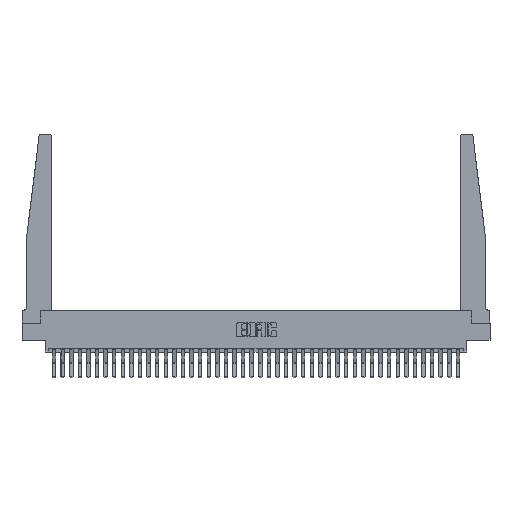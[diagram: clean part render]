
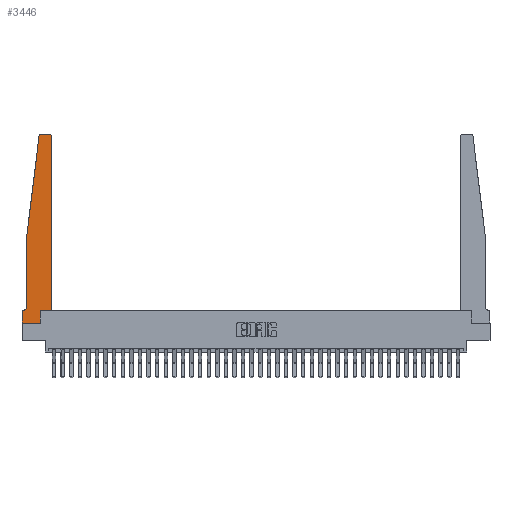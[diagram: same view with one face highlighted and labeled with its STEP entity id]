
A CAD part, top view. The second image highlights one B-rep face of the part: STEP entity #3446.
In plain terms, the highlighted planar face has unit normal (0, 0, 1).
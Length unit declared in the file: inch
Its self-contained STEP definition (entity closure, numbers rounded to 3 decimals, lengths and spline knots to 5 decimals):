
#540 = CARTESIAN_POINT ( 'NONE',  ( 0.27653, 2.75, 0.37 ) ) ;
#650 = ORIENTED_EDGE ( 'NONE', *, *, #20434, .T. ) ;
#983 = CARTESIAN_POINT ( 'NONE',  ( 0.25, 2.75, 0.37 ) ) ;
#1507 = LINE ( 'NONE', #15884, #22641 ) ;
#3208 = VERTEX_POINT ( 'NONE', #31765 ) ;
#3403 = VERTEX_POINT ( 'NONE', #35305 ) ;
#3446 = ADVANCED_FACE ( 'NONE', ( #24439 ), #34013, .T. ) ;
#3788 = LINE ( 'NONE', #25565, #17601 ) ;
#3988 = DIRECTION ( 'NONE',  ( 0., 1., 0. ) ) ;
#4056 = VERTEX_POINT ( 'NONE', #32637 ) ;
#4245 = DIRECTION ( 'NONE',  ( 0., 0., 1. ) ) ;
#4459 = EDGE_LOOP ( 'NONE', ( #25759, #8160, #12875, #28646, #28439, #14412, #33113, #16651, #10961, #32557, #8460, #650 ) ) ;
#5536 = EDGE_CURVE ( 'NONE', #4056, #25676, #3788, .T. ) ;
#5599 = DIRECTION ( 'NONE',  ( 1., 0., 0. ) ) ;
#6557 = LINE ( 'NONE', #22729, #34736 ) ;
#6653 = CARTESIAN_POINT ( 'NONE',  ( 0.395, 2.75, 0.37 ) ) ;
#6776 = EDGE_CURVE ( 'NONE', #15526, #3403, #23460, .T. ) ;
#6938 = VECTOR ( 'NONE', #19695, 39.37008 ) ;
#7162 = EDGE_CURVE ( 'NONE', #23891, #4056, #19611, .T. ) ;
#7681 = DIRECTION ( 'NONE',  ( 0., -1., 0. ) ) ;
#8160 = ORIENTED_EDGE ( 'NONE', *, *, #6776, .T. ) ;
#8460 = ORIENTED_EDGE ( 'NONE', *, *, #5536, .T. ) ;
#10553 = CARTESIAN_POINT ( 'NONE',  ( 0.395, 2.72, 0.37 ) ) ;
#10701 = VECTOR ( 'NONE', #24409, 39.37008 ) ;
#10736 = LINE ( 'NONE', #14856, #15462 ) ;
#10961 = ORIENTED_EDGE ( 'NONE', *, *, #34672, .T. ) ;
#11161 = EDGE_CURVE ( 'NONE', #18633, #24408, #19381, .T. ) ;
#11274 = DIRECTION ( 'NONE',  ( 0., 0., -1. ) ) ;
#11340 = DIRECTION ( 'NONE',  ( 1., 0., 0. ) ) ;
#11742 = CARTESIAN_POINT ( 'NONE',  ( 0.2605, 0., 0.37 ) ) ;
#11994 = DIRECTION ( 'NONE',  ( -1., 0., 0. ) ) ;
#12469 = EDGE_CURVE ( 'NONE', #23445, #20112, #1507, .T. ) ;
#12875 = ORIENTED_EDGE ( 'NONE', *, *, #27185, .T. ) ;
#12993 = VECTOR ( 'NONE', #19134, 39.37008 ) ;
#13334 = DIRECTION ( 'NONE',  ( 1., 0., 0. ) ) ;
#13800 = CARTESIAN_POINT ( 'NONE',  ( 0., 0.1875, 0.37 ) ) ;
#14283 = LINE ( 'NONE', #16962, #6938 ) ;
#14360 = AXIS2_PLACEMENT_3D ( 'NONE', #10553, #29613, #13334 ) ;
#14412 = ORIENTED_EDGE ( 'NONE', *, *, #16298, .T. ) ;
#14856 = CARTESIAN_POINT ( 'NONE',  ( 0.2605, 0.18, 0.37 ) ) ;
#15130 = AXIS2_PLACEMENT_3D ( 'NONE', #27582, #11274, #30314 ) ;
#15462 = VECTOR ( 'NONE', #3988, 39.37008 ) ;
#15526 = VERTEX_POINT ( 'NONE', #540 ) ;
#15884 = CARTESIAN_POINT ( 'NONE',  ( 0.065, 1.25, 0.37 ) ) ;
#16215 = CARTESIAN_POINT ( 'NONE',  ( 0.065, 1.25, 0.37 ) ) ;
#16298 = EDGE_CURVE ( 'NONE', #3208, #18633, #6557, .T. ) ;
#16651 = ORIENTED_EDGE ( 'NONE', *, *, #25173, .T. ) ;
#16883 = LINE ( 'NONE', #983, #23257 ) ;
#16962 = CARTESIAN_POINT ( 'NONE',  ( 0., 0., 0.37 ) ) ;
#17053 = CARTESIAN_POINT ( 'NONE',  ( 0.2605, 0.18, 0.37 ) ) ;
#17131 = LINE ( 'NONE', #16215, #10701 ) ;
#17601 = VECTOR ( 'NONE', #28289, 39.37008 ) ;
#18633 = VERTEX_POINT ( 'NONE', #13800 ) ;
#18900 = VERTEX_POINT ( 'NONE', #6653 ) ;
#19134 = DIRECTION ( 'NONE',  ( 0., -1., 0. ) ) ;
#19295 = CARTESIAN_POINT ( 'NONE',  ( 0., 0.1875, 0.37 ) ) ;
#19381 = LINE ( 'NONE', #32630, #12993 ) ;
#19611 = LINE ( 'NONE', #27644, #20467 ) ;
#19695 = DIRECTION ( 'NONE',  ( 1., 0., 0. ) ) ;
#20112 = VERTEX_POINT ( 'NONE', #20136 ) ;
#20136 = CARTESIAN_POINT ( 'NONE',  ( 0.065, 0.2375, 0.37 ) ) ;
#20434 = EDGE_CURVE ( 'NONE', #25676, #18900, #25776, .T. ) ;
#20467 = VECTOR ( 'NONE', #11340, 39.37008 ) ;
#20691 = CARTESIAN_POINT ( 'NONE',  ( 0.27653, 2.72, 0.37 ) ) ;
#21899 = CIRCLE ( 'NONE', #15130, 0.05 ) ;
#22029 = DIRECTION ( 'NONE',  ( 0., 0., 1. ) ) ;
#22641 = VECTOR ( 'NONE', #7681, 39.37008 ) ;
#22729 = CARTESIAN_POINT ( 'NONE',  ( 0.065, 0.1875, 0.37 ) ) ;
#22935 = AXIS2_PLACEMENT_3D ( 'NONE', #19295, #22029, #5599 ) ;
#23065 = DIRECTION ( 'NONE',  ( -1., 0., 0. ) ) ;
#23257 = VECTOR ( 'NONE', #23065, 39.37008 ) ;
#23428 = DIRECTION ( 'NONE',  ( 1., 0., 0. ) ) ;
#23445 = VERTEX_POINT ( 'NONE', #32107 ) ;
#23460 = CIRCLE ( 'NONE', #29601, 0.03 ) ;
#23891 = VERTEX_POINT ( 'NONE', #17053 ) ;
#24408 = VERTEX_POINT ( 'NONE', #29943 ) ;
#24409 = DIRECTION ( 'NONE',  ( -0.122, -0.992, 0. ) ) ;
#24439 = FACE_OUTER_BOUND ( 'NONE', #4459, .T. ) ;
#25173 = EDGE_CURVE ( 'NONE', #24408, #32678, #14283, .T. ) ;
#25565 = CARTESIAN_POINT ( 'NONE',  ( 0.425, 0.18, 0.37 ) ) ;
#25676 = VERTEX_POINT ( 'NONE', #32354 ) ;
#25759 = ORIENTED_EDGE ( 'NONE', *, *, #32772, .T. ) ;
#25776 = CIRCLE ( 'NONE', #14360, 0.03 ) ;
#25839 = EDGE_CURVE ( 'NONE', #20112, #3208, #21899, .T. ) ;
#27185 = EDGE_CURVE ( 'NONE', #3403, #23445, #17131, .T. ) ;
#27582 = CARTESIAN_POINT ( 'NONE',  ( 0.015, 0.2375, 0.37 ) ) ;
#27644 = CARTESIAN_POINT ( 'NONE',  ( 0.425, 0.18, 0.37 ) ) ;
#28289 = DIRECTION ( 'NONE',  ( 0., 1., 0. ) ) ;
#28439 = ORIENTED_EDGE ( 'NONE', *, *, #25839, .T. ) ;
#28646 = ORIENTED_EDGE ( 'NONE', *, *, #12469, .T. ) ;
#29601 = AXIS2_PLACEMENT_3D ( 'NONE', #20691, #4245, #23428 ) ;
#29613 = DIRECTION ( 'NONE',  ( 0., 0., 1. ) ) ;
#29943 = CARTESIAN_POINT ( 'NONE',  ( 0., 0., 0.37 ) ) ;
#30314 = DIRECTION ( 'NONE',  ( -1., 0., 0. ) ) ;
#31765 = CARTESIAN_POINT ( 'NONE',  ( 0.015, 0.1875, 0.37 ) ) ;
#32107 = CARTESIAN_POINT ( 'NONE',  ( 0.065, 1.25, 0.37 ) ) ;
#32354 = CARTESIAN_POINT ( 'NONE',  ( 0.425, 2.72, 0.37 ) ) ;
#32557 = ORIENTED_EDGE ( 'NONE', *, *, #7162, .T. ) ;
#32630 = CARTESIAN_POINT ( 'NONE',  ( 0., 0., 0.37 ) ) ;
#32637 = CARTESIAN_POINT ( 'NONE',  ( 0.425, 0.18, 0.37 ) ) ;
#32678 = VERTEX_POINT ( 'NONE', #11742 ) ;
#32772 = EDGE_CURVE ( 'NONE', #18900, #15526, #16883, .T. ) ;
#33113 = ORIENTED_EDGE ( 'NONE', *, *, #11161, .T. ) ;
#34013 = PLANE ( 'NONE',  #22935 ) ;
#34672 = EDGE_CURVE ( 'NONE', #32678, #23891, #10736, .T. ) ;
#34736 = VECTOR ( 'NONE', #11994, 39.37008 ) ;
#35305 = CARTESIAN_POINT ( 'NONE',  ( 0.24675, 2.72367, 0.37 ) ) ;
